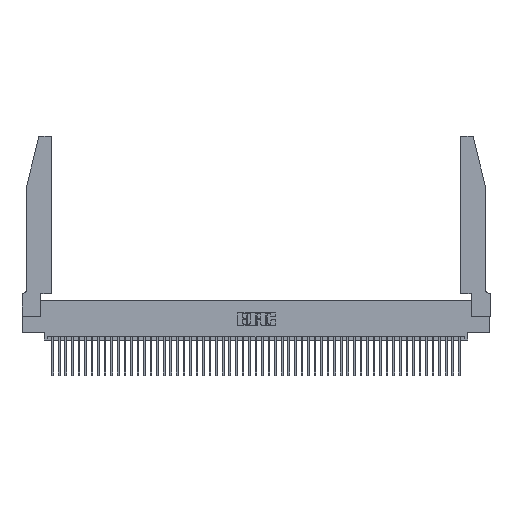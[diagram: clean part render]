
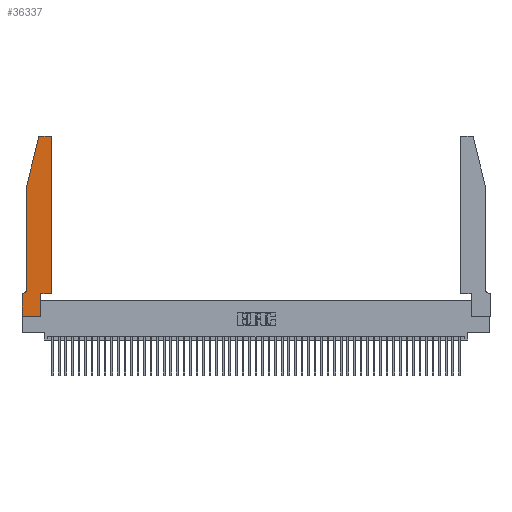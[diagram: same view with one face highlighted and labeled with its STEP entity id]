
A CAD part, top view. The second image highlights one B-rep face of the part: STEP entity #36337.
In plain terms, the highlighted planar face has unit normal (0, 0, 1).
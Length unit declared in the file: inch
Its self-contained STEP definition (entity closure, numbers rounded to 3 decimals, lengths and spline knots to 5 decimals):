
#212 = CARTESIAN_POINT ( 'NONE',  ( 0.2865, 0.35, 0.37 ) ) ;
#356 = VECTOR ( 'NONE', #21670, 39.37008 ) ;
#555 = LINE ( 'NONE', #47192, #16750 ) ;
#711 = DIRECTION ( 'NONE',  ( 1., 0., 0. ) ) ;
#1193 = CARTESIAN_POINT ( 'NONE',  ( 0.4505, 0.35, 0.37 ) ) ;
#1616 = ORIENTED_EDGE ( 'NONE', *, *, #44480, .T. ) ;
#1878 = ORIENTED_EDGE ( 'NONE', *, *, #29972, .T. ) ;
#1911 = VECTOR ( 'NONE', #27372, 39.37008 ) ;
#2599 = CIRCLE ( 'NONE', #44531, 0.03 ) ;
#3282 = VERTEX_POINT ( 'NONE', #10184 ) ;
#3789 = EDGE_CURVE ( 'NONE', #35162, #42435, #11193, .T. ) ;
#4114 = DIRECTION ( 'NONE',  ( 0., 0., 1. ) ) ;
#4828 = DIRECTION ( 'NONE',  ( 0., 0., 1. ) ) ;
#5177 = EDGE_CURVE ( 'NONE', #16930, #35162, #37278, .T. ) ;
#5778 = VERTEX_POINT ( 'NONE', #16544 ) ;
#5942 = EDGE_CURVE ( 'NONE', #17150, #5778, #43380, .T. ) ;
#6589 = EDGE_CURVE ( 'NONE', #20939, #16418, #32118, .T. ) ;
#6670 = VERTEX_POINT ( 'NONE', #29574 ) ;
#7754 = VECTOR ( 'NONE', #12243, 39.37008 ) ;
#8088 = DIRECTION ( 'NONE',  ( 1., 0., 0. ) ) ;
#8814 = CARTESIAN_POINT ( 'NONE',  ( 0., 0.35, 0.37 ) ) ;
#9170 = PLANE ( 'NONE',  #9963 ) ;
#9190 = ORIENTED_EDGE ( 'NONE', *, *, #3789, .T. ) ;
#9689 = CARTESIAN_POINT ( 'NONE',  ( 0.0755, 0.42, 0.37 ) ) ;
#9762 = VECTOR ( 'NONE', #37052, 39.37008 ) ;
#9963 = AXIS2_PLACEMENT_3D ( 'NONE', #8814, #4828, #32664 ) ;
#10184 = CARTESIAN_POINT ( 'NONE',  ( 0.0755, 2., 0.37 ) ) ;
#11193 = LINE ( 'NONE', #1193, #17479 ) ;
#11236 = CARTESIAN_POINT ( 'NONE',  ( 0.284, 2.75, 0.37 ) ) ;
#11747 = VECTOR ( 'NONE', #16063, 39.37008 ) ;
#12243 = DIRECTION ( 'NONE',  ( 0., 1., 0. ) ) ;
#12511 = DIRECTION ( 'NONE',  ( 0., 0., -1. ) ) ;
#12624 = CARTESIAN_POINT ( 'NONE',  ( 0., 0.35, 0.37 ) ) ;
#12886 = DIRECTION ( 'NONE',  ( 0., 0., 1. ) ) ;
#13229 = FACE_OUTER_BOUND ( 'NONE', #36322, .T. ) ;
#13674 = DIRECTION ( 'NONE',  ( -0.239, -0.971, 0. ) ) ;
#14353 = CARTESIAN_POINT ( 'NONE',  ( 0.0755, 2., 0.37 ) ) ;
#15825 = ORIENTED_EDGE ( 'NONE', *, *, #5177, .T. ) ;
#16015 = CARTESIAN_POINT ( 'NONE',  ( 0.0055, 0.42, 0.37 ) ) ;
#16063 = DIRECTION ( 'NONE',  ( 0., 1., 0. ) ) ;
#16418 = VERTEX_POINT ( 'NONE', #47800 ) ;
#16544 = CARTESIAN_POINT ( 'NONE',  ( 0., 0., 0.37 ) ) ;
#16750 = VECTOR ( 'NONE', #43365, 39.37008 ) ;
#16930 = VERTEX_POINT ( 'NONE', #50580 ) ;
#17150 = VERTEX_POINT ( 'NONE', #12624 ) ;
#17214 = DIRECTION ( 'NONE',  ( 1., 0., 0. ) ) ;
#17479 = VECTOR ( 'NONE', #17214, 39.37008 ) ;
#18844 = ORIENTED_EDGE ( 'NONE', *, *, #22493, .T. ) ;
#19642 = ORIENTED_EDGE ( 'NONE', *, *, #33761, .T. ) ;
#20939 = VERTEX_POINT ( 'NONE', #9689 ) ;
#20981 = ORIENTED_EDGE ( 'NONE', *, *, #26218, .T. ) ;
#21670 = DIRECTION ( 'NONE',  ( -1., 0., 0. ) ) ;
#21851 = CARTESIAN_POINT ( 'NONE',  ( 0.0755, 0.35, 0.37 ) ) ;
#22493 = EDGE_CURVE ( 'NONE', #50870, #41459, #2599, .T. ) ;
#24040 = LINE ( 'NONE', #21851, #356 ) ;
#24041 = CARTESIAN_POINT ( 'NONE',  ( 0.284, 2.72, 0.37 ) ) ;
#24218 = EDGE_CURVE ( 'NONE', #3282, #20939, #555, .T. ) ;
#24435 = CARTESIAN_POINT ( 'NONE',  ( 0.2865, 0.35, 0.37 ) ) ;
#24545 = DIRECTION ( 'NONE',  ( -1., 0., 0. ) ) ;
#24628 = EDGE_CURVE ( 'NONE', #5778, #16930, #48390, .T. ) ;
#26067 = LINE ( 'NONE', #14353, #44102 ) ;
#26218 = EDGE_CURVE ( 'NONE', #42435, #50870, #33309, .T. ) ;
#27335 = VERTEX_POINT ( 'NONE', #11236 ) ;
#27372 = DIRECTION ( 'NONE',  ( -1., 0., 0. ) ) ;
#27964 = CARTESIAN_POINT ( 'NONE',  ( 0.4205, 2.72, 0.37 ) ) ;
#29065 = CARTESIAN_POINT ( 'NONE',  ( 0., 0., 0.37 ) ) ;
#29574 = CARTESIAN_POINT ( 'NONE',  ( 0.25487, 2.72718, 0.37 ) ) ;
#29972 = EDGE_CURVE ( 'NONE', #41459, #27335, #42371, .T. ) ;
#31601 = VECTOR ( 'NONE', #34321, 39.37008 ) ;
#31749 = ORIENTED_EDGE ( 'NONE', *, *, #33453, .T. ) ;
#32118 = CIRCLE ( 'NONE', #47955, 0.07 ) ;
#32247 = CARTESIAN_POINT ( 'NONE',  ( 0.4505, 0.35, 0.37 ) ) ;
#32455 = CARTESIAN_POINT ( 'NONE',  ( 0.4205, 2.75, 0.37 ) ) ;
#32664 = DIRECTION ( 'NONE',  ( 1., 0., 0. ) ) ;
#32902 = AXIS2_PLACEMENT_3D ( 'NONE', #24041, #12886, #711 ) ;
#33309 = LINE ( 'NONE', #32247, #7754 ) ;
#33453 = EDGE_CURVE ( 'NONE', #16418, #17150, #24040, .T. ) ;
#33493 = CARTESIAN_POINT ( 'NONE',  ( 0.4505, 0.35, 0.37 ) ) ;
#33761 = EDGE_CURVE ( 'NONE', #27335, #6670, #42035, .T. ) ;
#34321 = DIRECTION ( 'NONE',  ( 1., 0., 0. ) ) ;
#34867 = ORIENTED_EDGE ( 'NONE', *, *, #6589, .T. ) ;
#35162 = VERTEX_POINT ( 'NONE', #24435 ) ;
#36322 = EDGE_LOOP ( 'NONE', ( #1878, #19642, #1616, #43940, #34867, #31749, #48851, #43044, #15825, #9190, #20981, #18844 ) ) ;
#36337 = ADVANCED_FACE ( 'NONE', ( #13229 ), #9170, .T. ) ;
#37052 = DIRECTION ( 'NONE',  ( 0., -1., 0. ) ) ;
#37278 = LINE ( 'NONE', #212, #11747 ) ;
#41459 = VERTEX_POINT ( 'NONE', #32455 ) ;
#42035 = CIRCLE ( 'NONE', #32902, 0.03 ) ;
#42371 = LINE ( 'NONE', #47676, #1911 ) ;
#42435 = VERTEX_POINT ( 'NONE', #33493 ) ;
#43044 = ORIENTED_EDGE ( 'NONE', *, *, #24628, .T. ) ;
#43365 = DIRECTION ( 'NONE',  ( 0., -1., 0. ) ) ;
#43380 = LINE ( 'NONE', #29065, #9762 ) ;
#43940 = ORIENTED_EDGE ( 'NONE', *, *, #24218, .T. ) ;
#44102 = VECTOR ( 'NONE', #13674, 39.37008 ) ;
#44480 = EDGE_CURVE ( 'NONE', #6670, #3282, #26067, .T. ) ;
#44531 = AXIS2_PLACEMENT_3D ( 'NONE', #27964, #4114, #8088 ) ;
#45731 = CARTESIAN_POINT ( 'NONE',  ( 0.4505, 2.72, 0.37 ) ) ;
#47192 = CARTESIAN_POINT ( 'NONE',  ( 0.0755, 2., 0.37 ) ) ;
#47676 = CARTESIAN_POINT ( 'NONE',  ( 0.2605, 2.75, 0.37 ) ) ;
#47800 = CARTESIAN_POINT ( 'NONE',  ( 0.0055, 0.35, 0.37 ) ) ;
#47955 = AXIS2_PLACEMENT_3D ( 'NONE', #16015, #12511, #24545 ) ;
#48390 = LINE ( 'NONE', #50684, #31601 ) ;
#48851 = ORIENTED_EDGE ( 'NONE', *, *, #5942, .T. ) ;
#50580 = CARTESIAN_POINT ( 'NONE',  ( 0.2865, 0., 0.37 ) ) ;
#50684 = CARTESIAN_POINT ( 'NONE',  ( 0., 0., 0.37 ) ) ;
#50870 = VERTEX_POINT ( 'NONE', #45731 ) ;
